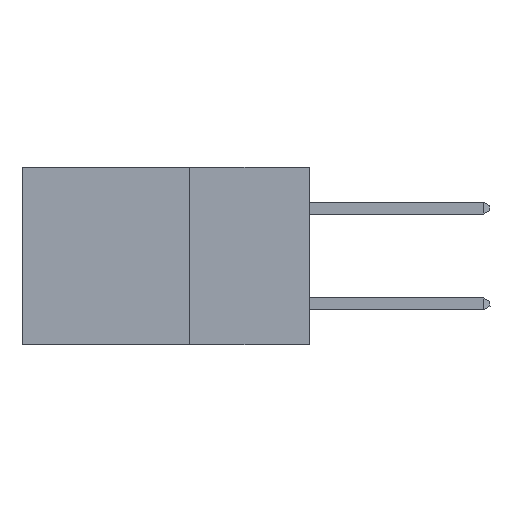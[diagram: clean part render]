
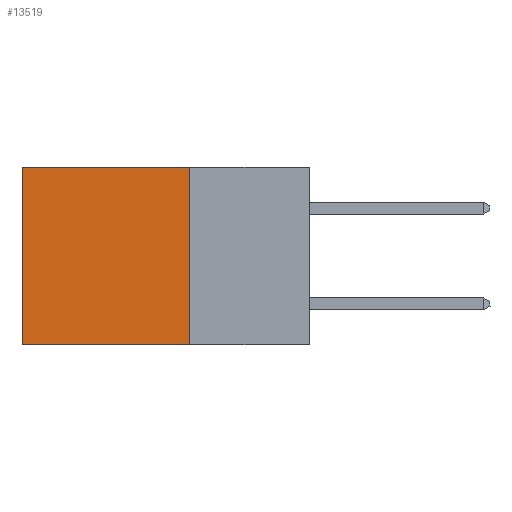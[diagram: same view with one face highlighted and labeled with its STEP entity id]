
A CAD part, left-side view. The second image highlights one B-rep face of the part: STEP entity #13519.
In plain terms, the highlighted planar face has unit normal (-1, 0, 0).
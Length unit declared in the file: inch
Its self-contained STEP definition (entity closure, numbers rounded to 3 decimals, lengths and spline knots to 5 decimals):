
#905 = EDGE_LOOP ( 'NONE', ( #5286, #18778, #14249, #18932 ) ) ;
#1609 = VECTOR ( 'NONE', #9243, 39.37008 ) ;
#2647 = PLANE ( 'NONE',  #16564 ) ;
#3112 = CARTESIAN_POINT ( 'NONE',  ( 0.2875, 0.6, -0.37 ) ) ;
#3436 = VECTOR ( 'NONE', #14295, 39.37008 ) ;
#3562 = CARTESIAN_POINT ( 'NONE',  ( 0.2875, 0.6, 0. ) ) ;
#4529 = CARTESIAN_POINT ( 'NONE',  ( 0.2875, 0.25, -0.37 ) ) ;
#4547 = CARTESIAN_POINT ( 'NONE',  ( 0.2875, 0.6, 0. ) ) ;
#5286 = ORIENTED_EDGE ( 'NONE', *, *, #6343, .T. ) ;
#5601 = LINE ( 'NONE', #4547, #16915 ) ;
#6193 = CARTESIAN_POINT ( 'NONE',  ( 0.2875, 0.25, 0. ) ) ;
#6250 = LINE ( 'NONE', #18540, #14523 ) ;
#6343 = EDGE_CURVE ( 'NONE', #18132, #15655, #5601, .T. ) ;
#6484 = LINE ( 'NONE', #18171, #1609 ) ;
#8507 = DIRECTION ( 'NONE',  ( 1., 0., 0. ) ) ;
#9243 = DIRECTION ( 'NONE',  ( 0., 1., 0. ) ) ;
#9607 = DIRECTION ( 'NONE',  ( 0., 0., -1. ) ) ;
#10543 = VERTEX_POINT ( 'NONE', #4529 ) ;
#11116 = LINE ( 'NONE', #12747, #3436 ) ;
#12747 = CARTESIAN_POINT ( 'NONE',  ( 0.2875, 0.25, 0. ) ) ;
#13222 = DIRECTION ( 'NONE',  ( 0., 0., -1. ) ) ;
#13519 = ADVANCED_FACE ( 'NONE', ( #18523 ), #2647, .F. ) ;
#13851 = EDGE_CURVE ( 'NONE', #10543, #15655, #6484, .T. ) ;
#14044 = EDGE_CURVE ( 'NONE', #16679, #10543, #6250, .T. ) ;
#14249 = ORIENTED_EDGE ( 'NONE', *, *, #14044, .F. ) ;
#14295 = DIRECTION ( 'NONE',  ( 0., 1., 0. ) ) ;
#14523 = VECTOR ( 'NONE', #9607, 39.37008 ) ;
#15655 = VERTEX_POINT ( 'NONE', #3112 ) ;
#16564 = AXIS2_PLACEMENT_3D ( 'NONE', #17394, #8507, #18858 ) ;
#16679 = VERTEX_POINT ( 'NONE', #6193 ) ;
#16915 = VECTOR ( 'NONE', #13222, 39.37008 ) ;
#17394 = CARTESIAN_POINT ( 'NONE',  ( 0.2875, 0.25, 0. ) ) ;
#17718 = EDGE_CURVE ( 'NONE', #16679, #18132, #11116, .T. ) ;
#18132 = VERTEX_POINT ( 'NONE', #3562 ) ;
#18171 = CARTESIAN_POINT ( 'NONE',  ( 0.2875, 0.25, -0.37 ) ) ;
#18523 = FACE_OUTER_BOUND ( 'NONE', #905, .T. ) ;
#18540 = CARTESIAN_POINT ( 'NONE',  ( 0.2875, 0.25, 0. ) ) ;
#18778 = ORIENTED_EDGE ( 'NONE', *, *, #13851, .F. ) ;
#18858 = DIRECTION ( 'NONE',  ( 0., 0., -1. ) ) ;
#18932 = ORIENTED_EDGE ( 'NONE', *, *, #17718, .T. ) ;
